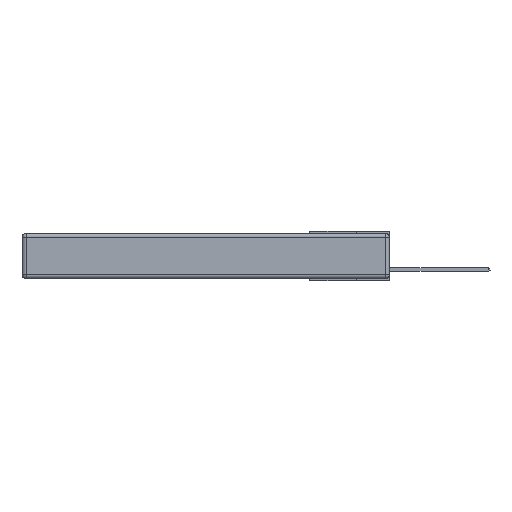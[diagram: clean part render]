
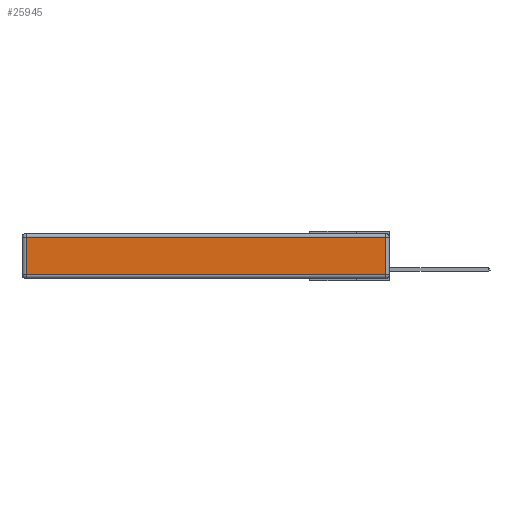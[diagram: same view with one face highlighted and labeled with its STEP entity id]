
A CAD part, left-side view. The second image highlights one B-rep face of the part: STEP entity #25945.
In plain terms, the highlighted planar face has unit normal (-1, 0, 0).
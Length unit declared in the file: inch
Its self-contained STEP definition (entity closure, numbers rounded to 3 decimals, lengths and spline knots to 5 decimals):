
#653 = CARTESIAN_POINT ( 'NONE',  ( 0., 2.72, -0.313 ) ) ;
#1085 = ORIENTED_EDGE ( 'NONE', *, *, #12407, .T. ) ;
#2623 = LINE ( 'NONE', #16538, #11329 ) ;
#3176 = VERTEX_POINT ( 'NONE', #8746 ) ;
#4308 = ORIENTED_EDGE ( 'NONE', *, *, #18768, .T. ) ;
#5271 = LINE ( 'NONE', #22572, #13649 ) ;
#6054 = DIRECTION ( 'NONE',  ( 0., 0., 1. ) ) ;
#6197 = VERTEX_POINT ( 'NONE', #22879 ) ;
#6572 = LINE ( 'NONE', #14599, #18553 ) ;
#8217 = DIRECTION ( 'NONE',  ( 0., 0., -1. ) ) ;
#8338 = VECTOR ( 'NONE', #6054, 39.37008 ) ;
#8746 = CARTESIAN_POINT ( 'NONE',  ( 0., 0.03, -0.03 ) ) ;
#10366 = DIRECTION ( 'NONE',  ( 0., 1., 0. ) ) ;
#10919 = FACE_OUTER_BOUND ( 'NONE', #23402, .T. ) ;
#11329 = VECTOR ( 'NONE', #8217, 39.37008 ) ;
#12193 = ORIENTED_EDGE ( 'NONE', *, *, #15810, .T. ) ;
#12229 = LINE ( 'NONE', #26596, #8338 ) ;
#12407 = EDGE_CURVE ( 'NONE', #16700, #6197, #6572, .T. ) ;
#12793 = DIRECTION ( 'NONE',  ( 0., 0., 1. ) ) ;
#12968 = CARTESIAN_POINT ( 'NONE',  ( 0., 0., -0.343 ) ) ;
#13062 = PLANE ( 'NONE',  #20408 ) ;
#13649 = VECTOR ( 'NONE', #10366, 39.37008 ) ;
#14304 = CARTESIAN_POINT ( 'NONE',  ( 0., 2.72, -0.03 ) ) ;
#14599 = CARTESIAN_POINT ( 'NONE',  ( 0., 0., -0.313 ) ) ;
#15810 = EDGE_CURVE ( 'NONE', #6197, #3176, #12229, .T. ) ;
#16538 = CARTESIAN_POINT ( 'NONE',  ( 0., 2.72, -0.343 ) ) ;
#16700 = VERTEX_POINT ( 'NONE', #653 ) ;
#18006 = VERTEX_POINT ( 'NONE', #14304 ) ;
#18553 = VECTOR ( 'NONE', #26585, 39.37008 ) ;
#18768 = EDGE_CURVE ( 'NONE', #3176, #18006, #5271, .T. ) ;
#19107 = DIRECTION ( 'NONE',  ( -1., 0., 0. ) ) ;
#19362 = ORIENTED_EDGE ( 'NONE', *, *, #20949, .T. ) ;
#20408 = AXIS2_PLACEMENT_3D ( 'NONE', #12968, #19107, #12793 ) ;
#20949 = EDGE_CURVE ( 'NONE', #18006, #16700, #2623, .T. ) ;
#22572 = CARTESIAN_POINT ( 'NONE',  ( 0., 2.75, -0.03 ) ) ;
#22879 = CARTESIAN_POINT ( 'NONE',  ( 0., 0.03, -0.313 ) ) ;
#23402 = EDGE_LOOP ( 'NONE', ( #1085, #12193, #4308, #19362 ) ) ;
#25945 = ADVANCED_FACE ( 'NONE', ( #10919 ), #13062, .T. ) ;
#26585 = DIRECTION ( 'NONE',  ( 0., -1., 0. ) ) ;
#26596 = CARTESIAN_POINT ( 'NONE',  ( 0., 0.03, -0.343 ) ) ;
